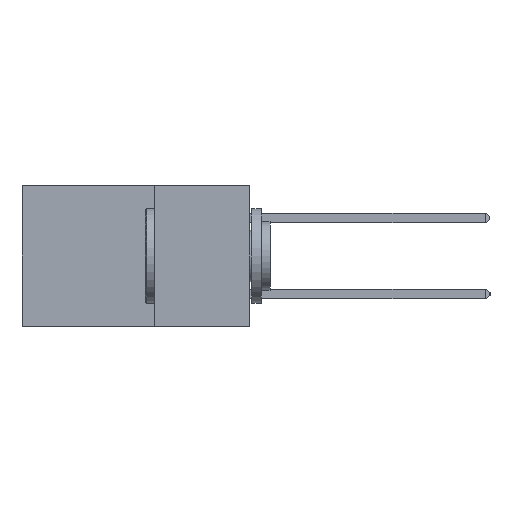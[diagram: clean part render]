
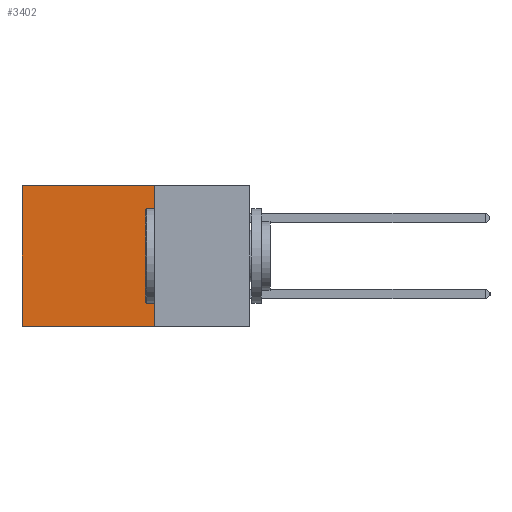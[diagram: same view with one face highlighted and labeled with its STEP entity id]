
A CAD part, left-side view. The second image highlights one B-rep face of the part: STEP entity #3402.
In plain terms, the highlighted planar face has unit normal (-1, 0, 0).
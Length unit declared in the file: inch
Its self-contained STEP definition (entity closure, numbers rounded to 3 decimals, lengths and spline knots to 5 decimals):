
#251 = VERTEX_POINT ( 'NONE', #5117 ) ;
#1115 = AXIS2_PLACEMENT_3D ( 'NONE', #12130, #8082, #1268 ) ;
#1116 = CARTESIAN_POINT ( 'NONE',  ( 0.2875, 0.6, -0.37 ) ) ;
#1268 = DIRECTION ( 'NONE',  ( 0., 0., -1. ) ) ;
#1843 = EDGE_CURVE ( 'NONE', #251, #5440, #11700, .T. ) ;
#2142 = FACE_OUTER_BOUND ( 'NONE', #3253, .T. ) ;
#2301 = VECTOR ( 'NONE', #12834, 39.37008 ) ;
#2404 = PLANE ( 'NONE',  #1115 ) ;
#2464 = LINE ( 'NONE', #8064, #10441 ) ;
#2638 = EDGE_CURVE ( 'NONE', #5440, #3005, #5721, .T. ) ;
#3005 = VERTEX_POINT ( 'NONE', #1116 ) ;
#3253 = EDGE_LOOP ( 'NONE', ( #11725, #13209, #13726, #10446 ) ) ;
#3402 = ADVANCED_FACE ( 'NONE', ( #2142 ), #2404, .F. ) ;
#5117 = CARTESIAN_POINT ( 'NONE',  ( 0.2875, 0.25, 0. ) ) ;
#5440 = VERTEX_POINT ( 'NONE', #6801 ) ;
#5460 = LINE ( 'NONE', #6717, #2301 ) ;
#5721 = LINE ( 'NONE', #6962, #8187 ) ;
#6717 = CARTESIAN_POINT ( 'NONE',  ( 0.2875, 0.25, 0. ) ) ;
#6801 = CARTESIAN_POINT ( 'NONE',  ( 0.2875, 0.25, -0.37 ) ) ;
#6873 = DIRECTION ( 'NONE',  ( 0., 1., 0. ) ) ;
#6962 = CARTESIAN_POINT ( 'NONE',  ( 0.2875, 0.25, -0.37 ) ) ;
#7786 = VERTEX_POINT ( 'NONE', #8188 ) ;
#8064 = CARTESIAN_POINT ( 'NONE',  ( 0.2875, 0.6, 0. ) ) ;
#8082 = DIRECTION ( 'NONE',  ( 1., 0., 0. ) ) ;
#8187 = VECTOR ( 'NONE', #6873, 39.37008 ) ;
#8188 = CARTESIAN_POINT ( 'NONE',  ( 0.2875, 0.6, 0. ) ) ;
#10441 = VECTOR ( 'NONE', #12152, 39.37008 ) ;
#10446 = ORIENTED_EDGE ( 'NONE', *, *, #12919, .T. ) ;
#11372 = VECTOR ( 'NONE', #11504, 39.37008 ) ;
#11504 = DIRECTION ( 'NONE',  ( 0., 0., -1. ) ) ;
#11700 = LINE ( 'NONE', #11874, #11372 ) ;
#11725 = ORIENTED_EDGE ( 'NONE', *, *, #13763, .T. ) ;
#11874 = CARTESIAN_POINT ( 'NONE',  ( 0.2875, 0.25, 0. ) ) ;
#12130 = CARTESIAN_POINT ( 'NONE',  ( 0.2875, 0.25, 0. ) ) ;
#12152 = DIRECTION ( 'NONE',  ( 0., 0., -1. ) ) ;
#12834 = DIRECTION ( 'NONE',  ( 0., 1., 0. ) ) ;
#12919 = EDGE_CURVE ( 'NONE', #251, #7786, #5460, .T. ) ;
#13209 = ORIENTED_EDGE ( 'NONE', *, *, #2638, .F. ) ;
#13726 = ORIENTED_EDGE ( 'NONE', *, *, #1843, .F. ) ;
#13763 = EDGE_CURVE ( 'NONE', #7786, #3005, #2464, .T. ) ;
